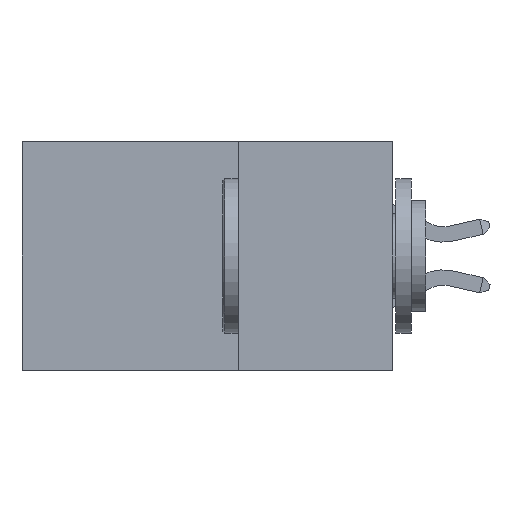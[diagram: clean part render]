
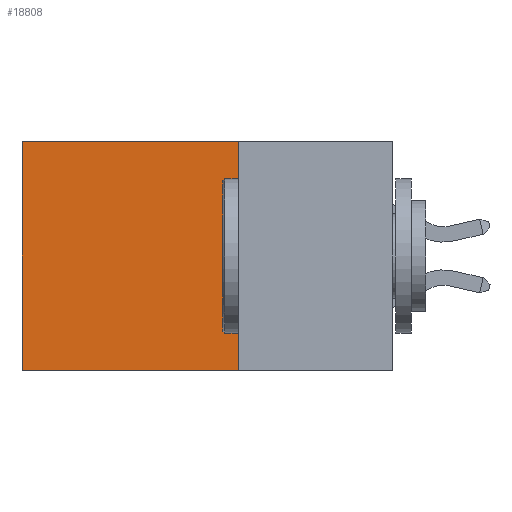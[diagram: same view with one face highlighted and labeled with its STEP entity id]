
A CAD part, left-side view. The second image highlights one B-rep face of the part: STEP entity #18808.
In plain terms, the highlighted planar face has unit normal (-1, 0, 0).
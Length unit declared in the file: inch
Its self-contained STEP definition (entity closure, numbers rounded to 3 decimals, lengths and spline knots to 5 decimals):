
#41 = VERTEX_POINT ( 'NONE', #22991 ) ;
#727 = LINE ( 'NONE', #3608, #14877 ) ;
#894 = CARTESIAN_POINT ( 'NONE',  ( 0.2875, 0.25, 0. ) ) ;
#1661 = DIRECTION ( 'NONE',  ( 1., 0., 0. ) ) ;
#3608 = CARTESIAN_POINT ( 'NONE',  ( 0.2875, 0.25, 0. ) ) ;
#3836 = EDGE_CURVE ( 'NONE', #41, #8835, #35482, .T. ) ;
#3967 = CARTESIAN_POINT ( 'NONE',  ( 0.2875, 0.25, 0. ) ) ;
#5244 = EDGE_LOOP ( 'NONE', ( #32664, #30953, #17481, #6457 ) ) ;
#6053 = PLANE ( 'NONE',  #9890 ) ;
#6457 = ORIENTED_EDGE ( 'NONE', *, *, #3836, .T. ) ;
#8835 = VERTEX_POINT ( 'NONE', #34716 ) ;
#9328 = CARTESIAN_POINT ( 'NONE',  ( 0.2875, 0.6, 0. ) ) ;
#9491 = VERTEX_POINT ( 'NONE', #17649 ) ;
#9890 = AXIS2_PLACEMENT_3D ( 'NONE', #894, #1661, #14271 ) ;
#12604 = EDGE_CURVE ( 'NONE', #9491, #12817, #26976, .T. ) ;
#12817 = VERTEX_POINT ( 'NONE', #24676 ) ;
#12826 = VECTOR ( 'NONE', #20171, 39.37008 ) ;
#14271 = DIRECTION ( 'NONE',  ( 0., 0., -1. ) ) ;
#14877 = VECTOR ( 'NONE', #26607, 39.37008 ) ;
#17481 = ORIENTED_EDGE ( 'NONE', *, *, #26567, .F. ) ;
#17649 = CARTESIAN_POINT ( 'NONE',  ( 0.2875, 0.25, -0.37 ) ) ;
#18808 = ADVANCED_FACE ( 'NONE', ( #27132 ), #6053, .F. ) ;
#19725 = EDGE_CURVE ( 'NONE', #8835, #12817, #33122, .T. ) ;
#20171 = DIRECTION ( 'NONE',  ( 0., 1., 0. ) ) ;
#22991 = CARTESIAN_POINT ( 'NONE',  ( 0.2875, 0.25, 0. ) ) ;
#24676 = CARTESIAN_POINT ( 'NONE',  ( 0.2875, 0.6, -0.37 ) ) ;
#26567 = EDGE_CURVE ( 'NONE', #41, #9491, #727, .T. ) ;
#26607 = DIRECTION ( 'NONE',  ( 0., 0., -1. ) ) ;
#26976 = LINE ( 'NONE', #31363, #12826 ) ;
#27132 = FACE_OUTER_BOUND ( 'NONE', #5244, .T. ) ;
#27486 = VECTOR ( 'NONE', #29687, 39.37008 ) ;
#29687 = DIRECTION ( 'NONE',  ( 0., 0., -1. ) ) ;
#30953 = ORIENTED_EDGE ( 'NONE', *, *, #12604, .F. ) ;
#31363 = CARTESIAN_POINT ( 'NONE',  ( 0.2875, 0.25, -0.37 ) ) ;
#32664 = ORIENTED_EDGE ( 'NONE', *, *, #19725, .T. ) ;
#33122 = LINE ( 'NONE', #9328, #27486 ) ;
#34559 = VECTOR ( 'NONE', #35009, 39.37008 ) ;
#34716 = CARTESIAN_POINT ( 'NONE',  ( 0.2875, 0.6, 0. ) ) ;
#35009 = DIRECTION ( 'NONE',  ( 0., 1., 0. ) ) ;
#35482 = LINE ( 'NONE', #3967, #34559 ) ;
